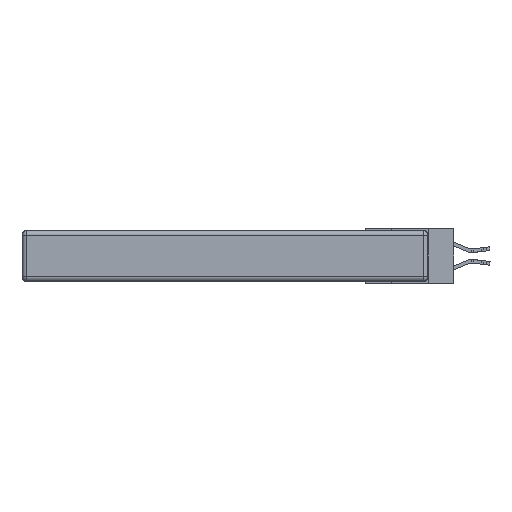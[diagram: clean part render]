
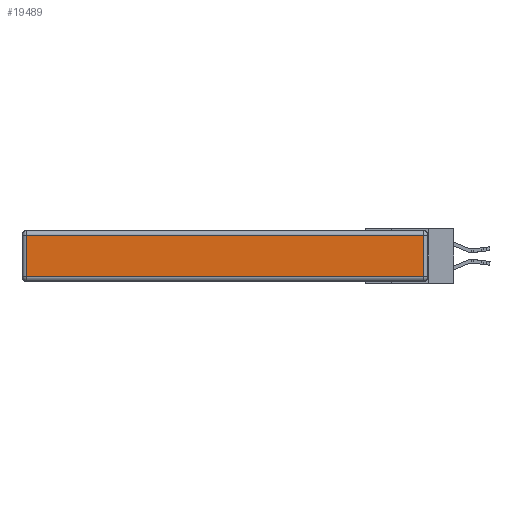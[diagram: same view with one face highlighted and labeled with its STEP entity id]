
A CAD part, left-side view. The second image highlights one B-rep face of the part: STEP entity #19489.
In plain terms, the highlighted planar face has unit normal (-1, 0, 0).
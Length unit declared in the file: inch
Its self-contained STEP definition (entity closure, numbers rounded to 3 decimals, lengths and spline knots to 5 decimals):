
#3001 = VERTEX_POINT ( 'NONE', #18079 ) ;
#3032 = EDGE_CURVE ( 'NONE', #4322, #15000, #27770, .T. ) ;
#4322 = VERTEX_POINT ( 'NONE', #15856 ) ;
#4471 = DIRECTION ( 'NONE',  ( 0., -1., 0. ) ) ;
#6848 = EDGE_LOOP ( 'NONE', ( #13036, #29808, #30823, #20128 ) ) ;
#7516 = CARTESIAN_POINT ( 'NONE',  ( 0., 2.72, -0.343 ) ) ;
#9067 = FACE_OUTER_BOUND ( 'NONE', #6848, .T. ) ;
#10410 = LINE ( 'NONE', #7516, #25374 ) ;
#10837 = LINE ( 'NONE', #31218, #19839 ) ;
#11841 = DIRECTION ( 'NONE',  ( 0., 1., 0. ) ) ;
#12312 = CARTESIAN_POINT ( 'NONE',  ( 0., 0.03, -0.343 ) ) ;
#12516 = AXIS2_PLACEMENT_3D ( 'NONE', #17045, #22309, #19911 ) ;
#13036 = ORIENTED_EDGE ( 'NONE', *, *, #3032, .T. ) ;
#13458 = EDGE_CURVE ( 'NONE', #3001, #28761, #10837, .T. ) ;
#15000 = VERTEX_POINT ( 'NONE', #17327 ) ;
#15856 = CARTESIAN_POINT ( 'NONE',  ( 0., 2.72, -0.313 ) ) ;
#17045 = CARTESIAN_POINT ( 'NONE',  ( 0., 0., -0.343 ) ) ;
#17327 = CARTESIAN_POINT ( 'NONE',  ( 0., 0.03, -0.313 ) ) ;
#18079 = CARTESIAN_POINT ( 'NONE',  ( 0., 0.03, -0.03 ) ) ;
#19489 = ADVANCED_FACE ( 'NONE', ( #9067 ), #25034, .T. ) ;
#19839 = VECTOR ( 'NONE', #11841, 39.37008 ) ;
#19911 = DIRECTION ( 'NONE',  ( 0., 0., 1. ) ) ;
#20128 = ORIENTED_EDGE ( 'NONE', *, *, #33058, .T. ) ;
#21319 = CARTESIAN_POINT ( 'NONE',  ( 0., 0., -0.313 ) ) ;
#22309 = DIRECTION ( 'NONE',  ( -1., 0., 0. ) ) ;
#23838 = EDGE_CURVE ( 'NONE', #15000, #3001, #31499, .T. ) ;
#25034 = PLANE ( 'NONE',  #12516 ) ;
#25161 = VECTOR ( 'NONE', #31309, 39.37008 ) ;
#25374 = VECTOR ( 'NONE', #31653, 39.37008 ) ;
#25637 = VECTOR ( 'NONE', #4471, 39.37008 ) ;
#27770 = LINE ( 'NONE', #21319, #25637 ) ;
#28237 = CARTESIAN_POINT ( 'NONE',  ( 0., 2.72, -0.03 ) ) ;
#28761 = VERTEX_POINT ( 'NONE', #28237 ) ;
#29808 = ORIENTED_EDGE ( 'NONE', *, *, #23838, .T. ) ;
#30823 = ORIENTED_EDGE ( 'NONE', *, *, #13458, .T. ) ;
#31218 = CARTESIAN_POINT ( 'NONE',  ( 0., 2.75, -0.03 ) ) ;
#31309 = DIRECTION ( 'NONE',  ( 0., 0., 1. ) ) ;
#31499 = LINE ( 'NONE', #12312, #25161 ) ;
#31653 = DIRECTION ( 'NONE',  ( 0., 0., -1. ) ) ;
#33058 = EDGE_CURVE ( 'NONE', #28761, #4322, #10410, .T. ) ;
